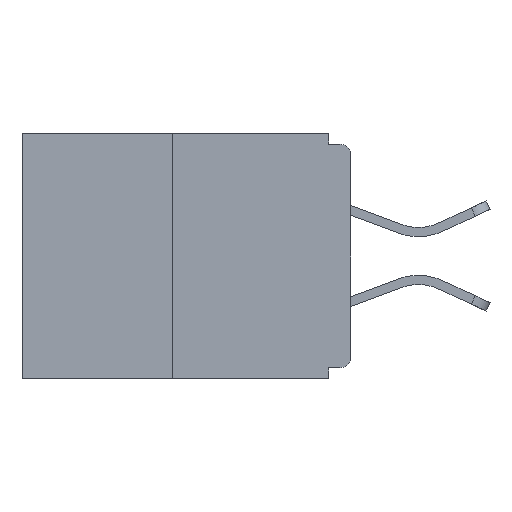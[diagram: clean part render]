
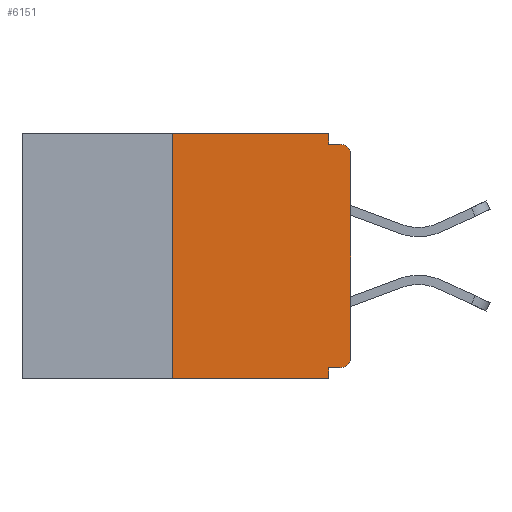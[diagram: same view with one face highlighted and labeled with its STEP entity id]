
A CAD part, left-side view. The second image highlights one B-rep face of the part: STEP entity #6151.
In plain terms, the highlighted planar face has unit normal (-1, 0, 0).
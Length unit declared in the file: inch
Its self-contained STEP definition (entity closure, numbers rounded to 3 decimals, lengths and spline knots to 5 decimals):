
#279 = EDGE_LOOP ( 'NONE', ( #25833, #9695, #10581, #14865, #16458, #23245, #14008, #14397, #13857, #20865 ) ) ;
#856 = DIRECTION ( 'NONE',  ( 0., 0., -1. ) ) ;
#1473 = LINE ( 'NONE', #20484, #6959 ) ;
#1555 = CARTESIAN_POINT ( 'NONE',  ( 0., 0.25, 0. ) ) ;
#1683 = VECTOR ( 'NONE', #20770, 39.37008 ) ;
#1776 = AXIS2_PLACEMENT_3D ( 'NONE', #23897, #11553, #856 ) ;
#2188 = LINE ( 'NONE', #22492, #7989 ) ;
#2944 = FACE_OUTER_BOUND ( 'NONE', #279, .T. ) ;
#3087 = VERTEX_POINT ( 'NONE', #11665 ) ;
#3274 = VERTEX_POINT ( 'NONE', #21323 ) ;
#3510 = DIRECTION ( 'NONE',  ( 0., 0., -1. ) ) ;
#3839 = EDGE_CURVE ( 'NONE', #19755, #10415, #22025, .T. ) ;
#4312 = CIRCLE ( 'NONE', #18896, 0.015 ) ;
#4387 = EDGE_CURVE ( 'NONE', #5073, #3087, #4312, .T. ) ;
#4528 = VERTEX_POINT ( 'NONE', #18900 ) ;
#5073 = VERTEX_POINT ( 'NONE', #24297 ) ;
#5572 = DIRECTION ( 'NONE',  ( 1., 0., 0. ) ) ;
#5575 = VECTOR ( 'NONE', #19903, 39.37008 ) ;
#5914 = VECTOR ( 'NONE', #19777, 39.37008 ) ;
#6151 = ADVANCED_FACE ( 'NONE', ( #2944 ), #19362, .F. ) ;
#6189 = VECTOR ( 'NONE', #24821, 39.37008 ) ;
#6959 = VECTOR ( 'NONE', #16791, 39.37008 ) ;
#7519 = LINE ( 'NONE', #13420, #5914 ) ;
#7989 = VECTOR ( 'NONE', #10528, 39.37008 ) ;
#8356 = VERTEX_POINT ( 'NONE', #11756 ) ;
#8673 = CARTESIAN_POINT ( 'NONE',  ( 0., 0.46, -0.343 ) ) ;
#8888 = CARTESIAN_POINT ( 'NONE',  ( 0., 0.031, -0.328 ) ) ;
#8905 = EDGE_CURVE ( 'NONE', #19768, #8356, #14037, .T. ) ;
#9167 = CARTESIAN_POINT ( 'NONE',  ( 0., 0., -0.313 ) ) ;
#9695 = ORIENTED_EDGE ( 'NONE', *, *, #3839, .F. ) ;
#10415 = VERTEX_POINT ( 'NONE', #1555 ) ;
#10417 = LINE ( 'NONE', #8673, #1683 ) ;
#10528 = DIRECTION ( 'NONE',  ( 0., 0., -1. ) ) ;
#10581 = ORIENTED_EDGE ( 'NONE', *, *, #18424, .T. ) ;
#11553 = DIRECTION ( 'NONE',  ( -1., 0., 0. ) ) ;
#11665 = CARTESIAN_POINT ( 'NONE',  ( 0., 0.015, -0.015 ) ) ;
#11756 = CARTESIAN_POINT ( 'NONE',  ( 0., 0.031, -0.343 ) ) ;
#12070 = EDGE_CURVE ( 'NONE', #4528, #13996, #2188, .T. ) ;
#12643 = DIRECTION ( 'NONE',  ( 0., 0., -1. ) ) ;
#12837 = VERTEX_POINT ( 'NONE', #9167 ) ;
#13328 = EDGE_CURVE ( 'NONE', #13996, #3087, #1473, .T. ) ;
#13420 = CARTESIAN_POINT ( 'NONE',  ( 0., 0., 0. ) ) ;
#13857 = ORIENTED_EDGE ( 'NONE', *, *, #13328, .F. ) ;
#13871 = VECTOR ( 'NONE', #23409, 39.37008 ) ;
#13996 = VERTEX_POINT ( 'NONE', #14302 ) ;
#14008 = ORIENTED_EDGE ( 'NONE', *, *, #14972, .T. ) ;
#14037 = LINE ( 'NONE', #24969, #26322 ) ;
#14302 = CARTESIAN_POINT ( 'NONE',  ( 0., 0.031, -0.015 ) ) ;
#14397 = ORIENTED_EDGE ( 'NONE', *, *, #4387, .T. ) ;
#14518 = LINE ( 'NONE', #21312, #13871 ) ;
#14865 = ORIENTED_EDGE ( 'NONE', *, *, #8905, .F. ) ;
#14972 = EDGE_CURVE ( 'NONE', #12837, #5073, #7519, .T. ) ;
#14977 = CARTESIAN_POINT ( 'NONE',  ( 0., 0.25, -0.343 ) ) ;
#15223 = CIRCLE ( 'NONE', #1776, 0.015 ) ;
#16458 = ORIENTED_EDGE ( 'NONE', *, *, #19520, .F. ) ;
#16791 = DIRECTION ( 'NONE',  ( 0., -1., 0. ) ) ;
#17724 = CARTESIAN_POINT ( 'NONE',  ( 0., 0.25, 0. ) ) ;
#18424 = EDGE_CURVE ( 'NONE', #19755, #8356, #10417, .T. ) ;
#18896 = AXIS2_PLACEMENT_3D ( 'NONE', #22909, #25020, #12643 ) ;
#18900 = CARTESIAN_POINT ( 'NONE',  ( 0., 0.031, 0. ) ) ;
#19033 = DIRECTION ( 'NONE',  ( 0., 0., -1. ) ) ;
#19362 = PLANE ( 'NONE',  #23439 ) ;
#19520 = EDGE_CURVE ( 'NONE', #3274, #19768, #14518, .T. ) ;
#19755 = VERTEX_POINT ( 'NONE', #14977 ) ;
#19768 = VERTEX_POINT ( 'NONE', #8888 ) ;
#19777 = DIRECTION ( 'NONE',  ( 0., 0., 1. ) ) ;
#19903 = DIRECTION ( 'NONE',  ( 0., 0., 1. ) ) ;
#20484 = CARTESIAN_POINT ( 'NONE',  ( 0., 0., -0.015 ) ) ;
#20770 = DIRECTION ( 'NONE',  ( 0., -1., 0. ) ) ;
#20865 = ORIENTED_EDGE ( 'NONE', *, *, #12070, .F. ) ;
#21039 = EDGE_CURVE ( 'NONE', #3274, #12837, #15223, .T. ) ;
#21312 = CARTESIAN_POINT ( 'NONE',  ( 0., 0., -0.328 ) ) ;
#21323 = CARTESIAN_POINT ( 'NONE',  ( 0., 0.015, -0.328 ) ) ;
#21349 = EDGE_CURVE ( 'NONE', #10415, #4528, #22315, .T. ) ;
#21788 = CARTESIAN_POINT ( 'NONE',  ( 0., 0.46, 0. ) ) ;
#22025 = LINE ( 'NONE', #17724, #5575 ) ;
#22315 = LINE ( 'NONE', #23161, #6189 ) ;
#22492 = CARTESIAN_POINT ( 'NONE',  ( 0., 0.031, 0. ) ) ;
#22909 = CARTESIAN_POINT ( 'NONE',  ( 0., 0.015, -0.03 ) ) ;
#23161 = CARTESIAN_POINT ( 'NONE',  ( 0., 0.46, 0. ) ) ;
#23245 = ORIENTED_EDGE ( 'NONE', *, *, #21039, .T. ) ;
#23409 = DIRECTION ( 'NONE',  ( 0., 1., 0. ) ) ;
#23439 = AXIS2_PLACEMENT_3D ( 'NONE', #21788, #5572, #3510 ) ;
#23897 = CARTESIAN_POINT ( 'NONE',  ( 0., 0.015, -0.313 ) ) ;
#24297 = CARTESIAN_POINT ( 'NONE',  ( 0., 0., -0.03 ) ) ;
#24821 = DIRECTION ( 'NONE',  ( 0., -1., 0. ) ) ;
#24969 = CARTESIAN_POINT ( 'NONE',  ( 0., 0.031, -0.343 ) ) ;
#25020 = DIRECTION ( 'NONE',  ( -1., 0., 0. ) ) ;
#25833 = ORIENTED_EDGE ( 'NONE', *, *, #21349, .F. ) ;
#26322 = VECTOR ( 'NONE', #19033, 39.37008 ) ;
